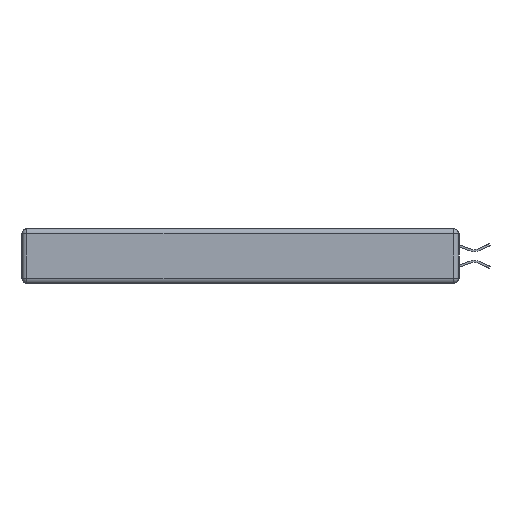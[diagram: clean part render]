
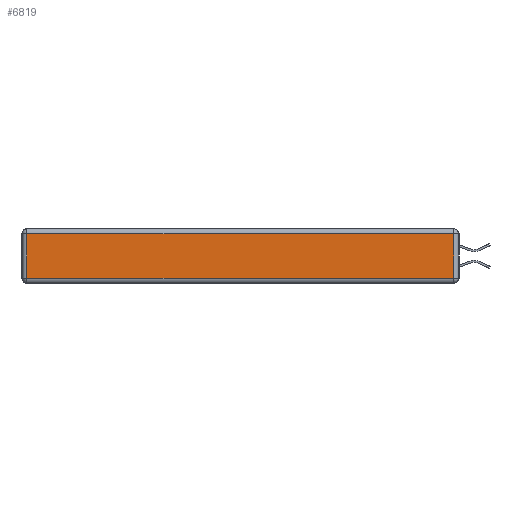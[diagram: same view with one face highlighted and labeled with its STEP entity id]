
A CAD part, left-side view. The second image highlights one B-rep face of the part: STEP entity #6819.
In plain terms, the highlighted planar face has unit normal (-1, 0, 0).
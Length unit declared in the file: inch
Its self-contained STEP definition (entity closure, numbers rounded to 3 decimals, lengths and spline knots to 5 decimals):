
#168 = EDGE_CURVE ( 'NONE', #13342, #15380, #3253, .T. ) ;
#256 = DIRECTION ( 'NONE',  ( 0., 1., 0. ) ) ;
#871 = FACE_OUTER_BOUND ( 'NONE', #8896, .T. ) ;
#1639 = DIRECTION ( 'NONE',  ( 0., 0., 1. ) ) ;
#2884 = CARTESIAN_POINT ( 'NONE',  ( 0., 2.72, -0.313 ) ) ;
#2909 = VERTEX_POINT ( 'NONE', #30069 ) ;
#2972 = ORIENTED_EDGE ( 'NONE', *, *, #168, .T. ) ;
#3253 = LINE ( 'NONE', #17547, #3682 ) ;
#3469 = VECTOR ( 'NONE', #16834, 39.37008 ) ;
#3682 = VECTOR ( 'NONE', #9636, 39.37008 ) ;
#4402 = EDGE_CURVE ( 'NONE', #2909, #6270, #30938, .T. ) ;
#5552 = CARTESIAN_POINT ( 'NONE',  ( 0., 2.75, -0.03 ) ) ;
#5843 = CARTESIAN_POINT ( 'NONE',  ( 0., 2.72, -0.03 ) ) ;
#6270 = VERTEX_POINT ( 'NONE', #15032 ) ;
#6819 = ADVANCED_FACE ( 'NONE', ( #871 ), #33113, .T. ) ;
#8307 = VECTOR ( 'NONE', #17777, 39.37008 ) ;
#8896 = EDGE_LOOP ( 'NONE', ( #13277, #34000, #28426, #2972 ) ) ;
#9636 = DIRECTION ( 'NONE',  ( 0., 0., -1. ) ) ;
#10080 = EDGE_CURVE ( 'NONE', #6270, #13342, #13976, .T. ) ;
#13277 = ORIENTED_EDGE ( 'NONE', *, *, #22836, .T. ) ;
#13342 = VERTEX_POINT ( 'NONE', #5843 ) ;
#13976 = LINE ( 'NONE', #5552, #18860 ) ;
#15032 = CARTESIAN_POINT ( 'NONE',  ( 0., 0.03, -0.03 ) ) ;
#15380 = VERTEX_POINT ( 'NONE', #2884 ) ;
#16834 = DIRECTION ( 'NONE',  ( 0., -1., 0. ) ) ;
#17547 = CARTESIAN_POINT ( 'NONE',  ( 0., 2.72, -0.343 ) ) ;
#17707 = DIRECTION ( 'NONE',  ( -1., 0., 0. ) ) ;
#17777 = DIRECTION ( 'NONE',  ( 0., 0., 1. ) ) ;
#18269 = LINE ( 'NONE', #32683, #3469 ) ;
#18860 = VECTOR ( 'NONE', #256, 39.37008 ) ;
#22836 = EDGE_CURVE ( 'NONE', #15380, #2909, #18269, .T. ) ;
#26064 = CARTESIAN_POINT ( 'NONE',  ( 0., 0.03, -0.343 ) ) ;
#28426 = ORIENTED_EDGE ( 'NONE', *, *, #10080, .T. ) ;
#29091 = AXIS2_PLACEMENT_3D ( 'NONE', #33461, #17707, #1639 ) ;
#30069 = CARTESIAN_POINT ( 'NONE',  ( 0., 0.03, -0.313 ) ) ;
#30938 = LINE ( 'NONE', #26064, #8307 ) ;
#32683 = CARTESIAN_POINT ( 'NONE',  ( 0., 0., -0.313 ) ) ;
#33113 = PLANE ( 'NONE',  #29091 ) ;
#33461 = CARTESIAN_POINT ( 'NONE',  ( 0., 0., -0.343 ) ) ;
#34000 = ORIENTED_EDGE ( 'NONE', *, *, #4402, .T. ) ;
